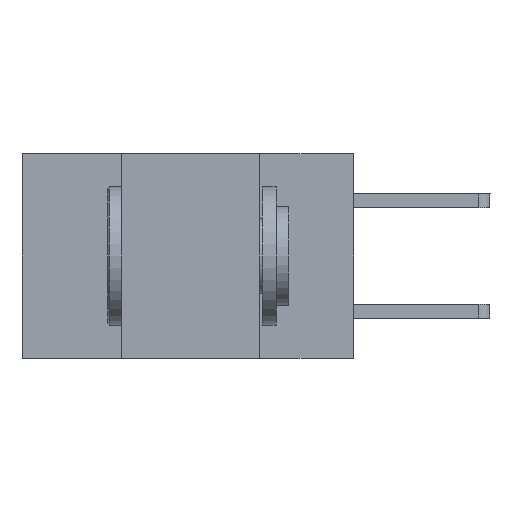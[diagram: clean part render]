
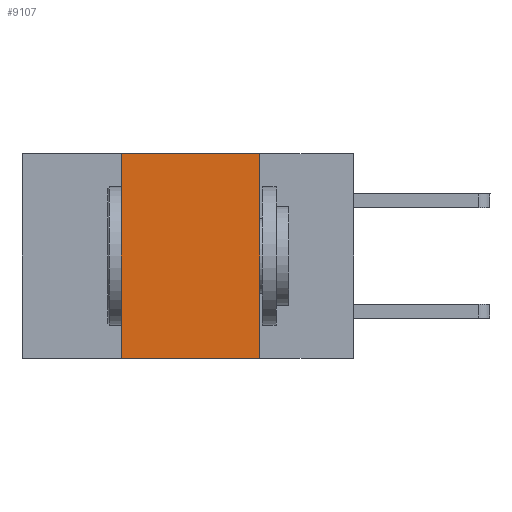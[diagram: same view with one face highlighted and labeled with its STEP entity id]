
A CAD part, left-side view. The second image highlights one B-rep face of the part: STEP entity #9107.
In plain terms, the highlighted planar face has unit normal (-1, 0, 0).
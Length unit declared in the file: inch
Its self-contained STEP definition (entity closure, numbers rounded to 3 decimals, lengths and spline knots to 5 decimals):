
#132 = ORIENTED_EDGE ( 'NONE', *, *, #9999, .F. ) ;
#559 = CARTESIAN_POINT ( 'NONE',  ( 0., 0.6, 0. ) ) ;
#1026 = VECTOR ( 'NONE', #10203, 39.37008 ) ;
#1145 = DIRECTION ( 'NONE',  ( 0., 0., -1. ) ) ;
#1267 = LINE ( 'NONE', #10129, #1026 ) ;
#1331 = DIRECTION ( 'NONE',  ( 0., -1., 0. ) ) ;
#1416 = PLANE ( 'NONE',  #8339 ) ;
#1461 = EDGE_CURVE ( 'NONE', #5429, #7339, #8008, .T. ) ;
#1601 = EDGE_CURVE ( 'NONE', #5429, #3258, #7479, .T. ) ;
#1764 = ORIENTED_EDGE ( 'NONE', *, *, #1461, .F. ) ;
#2212 = DIRECTION ( 'NONE',  ( 0., 0., -1. ) ) ;
#2246 = DIRECTION ( 'NONE',  ( 1., 0., 0. ) ) ;
#2762 = VECTOR ( 'NONE', #1331, 39.37008 ) ;
#3258 = VERTEX_POINT ( 'NONE', #4690 ) ;
#3493 = DIRECTION ( 'NONE',  ( 0., 0., 1. ) ) ;
#4401 = CARTESIAN_POINT ( 'NONE',  ( 0., 0.42, -0.37 ) ) ;
#4466 = EDGE_CURVE ( 'NONE', #6503, #3258, #9139, .T. ) ;
#4690 = CARTESIAN_POINT ( 'NONE',  ( 0., 0.17, -0.37 ) ) ;
#5098 = ORIENTED_EDGE ( 'NONE', *, *, #1601, .T. ) ;
#5429 = VERTEX_POINT ( 'NONE', #4401 ) ;
#6017 = CARTESIAN_POINT ( 'NONE',  ( 0., 0.6, -0.37 ) ) ;
#6081 = VECTOR ( 'NONE', #1145, 39.37008 ) ;
#6503 = VERTEX_POINT ( 'NONE', #8997 ) ;
#7046 = EDGE_LOOP ( 'NONE', ( #8940, #132, #1764, #5098 ) ) ;
#7339 = VERTEX_POINT ( 'NONE', #9498 ) ;
#7394 = CARTESIAN_POINT ( 'NONE',  ( 0., 0.42, 0. ) ) ;
#7479 = LINE ( 'NONE', #6017, #2762 ) ;
#7989 = FACE_OUTER_BOUND ( 'NONE', #7046, .T. ) ;
#8008 = LINE ( 'NONE', #7394, #9254 ) ;
#8339 = AXIS2_PLACEMENT_3D ( 'NONE', #559, #2246, #2212 ) ;
#8361 = CARTESIAN_POINT ( 'NONE',  ( 0., 0.17, 0. ) ) ;
#8940 = ORIENTED_EDGE ( 'NONE', *, *, #4466, .F. ) ;
#8997 = CARTESIAN_POINT ( 'NONE',  ( 0., 0.17, 0. ) ) ;
#9107 = ADVANCED_FACE ( 'NONE', ( #7989 ), #1416, .F. ) ;
#9139 = LINE ( 'NONE', #8361, #6081 ) ;
#9254 = VECTOR ( 'NONE', #3493, 39.37008 ) ;
#9498 = CARTESIAN_POINT ( 'NONE',  ( 0., 0.42, 0. ) ) ;
#9999 = EDGE_CURVE ( 'NONE', #7339, #6503, #1267, .T. ) ;
#10129 = CARTESIAN_POINT ( 'NONE',  ( 0., 0.6, 0. ) ) ;
#10203 = DIRECTION ( 'NONE',  ( 0., -1., 0. ) ) ;
